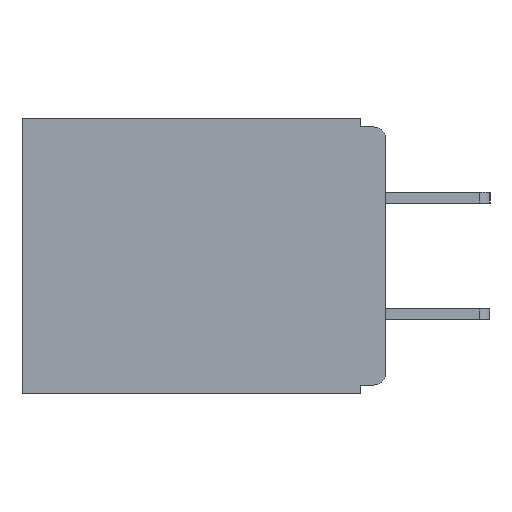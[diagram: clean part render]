
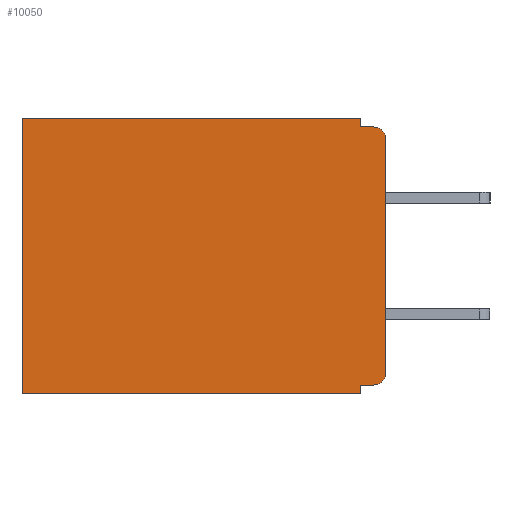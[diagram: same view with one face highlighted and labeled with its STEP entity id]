
A CAD part, left-side view. The second image highlights one B-rep face of the part: STEP entity #10050.
In plain terms, the highlighted planar face has unit normal (-1, 0, 0).
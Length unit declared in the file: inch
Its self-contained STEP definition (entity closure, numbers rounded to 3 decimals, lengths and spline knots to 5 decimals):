
#286 = LINE ( 'NONE', #6768, #24448 ) ;
#321 = DIRECTION ( 'NONE',  ( 0., 1., 0. ) ) ;
#664 = CARTESIAN_POINT ( 'NONE',  ( 0.3, 0., -0.33 ) ) ;
#1757 = CARTESIAN_POINT ( 'NONE',  ( 0.3, 0., -0.01 ) ) ;
#1906 = DIRECTION ( 'NONE',  ( 1., 0., 0. ) ) ;
#2193 = CARTESIAN_POINT ( 'NONE',  ( 0.3, 0.031, -0.32 ) ) ;
#2495 = LINE ( 'NONE', #664, #7075 ) ;
#2692 = DIRECTION ( 'NONE',  ( 0., 0., -1. ) ) ;
#2815 = CARTESIAN_POINT ( 'NONE',  ( 0.3, 0.437, -0.33 ) ) ;
#3931 = DIRECTION ( 'NONE',  ( 0., 0., -1. ) ) ;
#4431 = VECTOR ( 'NONE', #19743, 39.37008 ) ;
#6627 = CARTESIAN_POINT ( 'NONE',  ( 0.3, 0.015, -0.32 ) ) ;
#6768 = CARTESIAN_POINT ( 'NONE',  ( 0.3, 0., -0.33 ) ) ;
#7075 = VECTOR ( 'NONE', #2692, 39.37008 ) ;
#7215 = ORIENTED_EDGE ( 'NONE', *, *, #11535, .F. ) ;
#7394 = VECTOR ( 'NONE', #9188, 39.37008 ) ;
#7832 = EDGE_CURVE ( 'NONE', #14480, #10644, #13323, .T. ) ;
#7891 = VECTOR ( 'NONE', #321, 39.37008 ) ;
#8687 = DIRECTION ( 'NONE',  ( 0., 1., 0. ) ) ;
#9079 = VERTEX_POINT ( 'NONE', #23407 ) ;
#9143 = AXIS2_PLACEMENT_3D ( 'NONE', #13459, #1906, #15392 ) ;
#9188 = DIRECTION ( 'NONE',  ( 0., 0., -1. ) ) ;
#9227 = EDGE_CURVE ( 'NONE', #20354, #9079, #17417, .T. ) ;
#9714 = CARTESIAN_POINT ( 'NONE',  ( 0.3, 0.437, 0. ) ) ;
#10050 = ADVANCED_FACE ( 'NONE', ( #20315 ), #22793, .F. ) ;
#10409 = CARTESIAN_POINT ( 'NONE',  ( 0.3, 0., 0. ) ) ;
#10644 = VERTEX_POINT ( 'NONE', #9714 ) ;
#10676 = CARTESIAN_POINT ( 'NONE',  ( 0.3, 0.015, -0.305 ) ) ;
#10897 = LINE ( 'NONE', #11620, #20394 ) ;
#11111 = CARTESIAN_POINT ( 'NONE',  ( 0.3, 0.015, -0.025 ) ) ;
#11207 = VERTEX_POINT ( 'NONE', #22508 ) ;
#11514 = ORIENTED_EDGE ( 'NONE', *, *, #14341, .T. ) ;
#11535 = EDGE_CURVE ( 'NONE', #20855, #21771, #14666, .T. ) ;
#11620 = CARTESIAN_POINT ( 'NONE',  ( 0.3, 0.437, -0.33 ) ) ;
#11855 = EDGE_CURVE ( 'NONE', #18070, #24520, #23090, .T. ) ;
#12035 = CARTESIAN_POINT ( 'NONE',  ( 0.3, 0., -0.32 ) ) ;
#12287 = CARTESIAN_POINT ( 'NONE',  ( 0.3, 0.031, -0.33 ) ) ;
#12364 = DIRECTION ( 'NONE',  ( 0., 1., 0. ) ) ;
#12646 = DIRECTION ( 'NONE',  ( 0., 0., -1. ) ) ;
#12737 = VECTOR ( 'NONE', #12364, 39.37008 ) ;
#12825 = EDGE_CURVE ( 'NONE', #14480, #11207, #23047, .T. ) ;
#13076 = DIRECTION ( 'NONE',  ( 0., 0., -1. ) ) ;
#13110 = VECTOR ( 'NONE', #24518, 39.37008 ) ;
#13323 = LINE ( 'NONE', #10409, #12737 ) ;
#13459 = CARTESIAN_POINT ( 'NONE',  ( 0.3, 0., -0.33 ) ) ;
#14123 = ORIENTED_EDGE ( 'NONE', *, *, #14417, .F. ) ;
#14160 = CARTESIAN_POINT ( 'NONE',  ( 0.3, 0., -0.025 ) ) ;
#14341 = EDGE_CURVE ( 'NONE', #10644, #20374, #10897, .T. ) ;
#14417 = EDGE_CURVE ( 'NONE', #20354, #20855, #22397, .T. ) ;
#14480 = VERTEX_POINT ( 'NONE', #15953 ) ;
#14666 = LINE ( 'NONE', #17859, #4431 ) ;
#14939 = CARTESIAN_POINT ( 'NONE',  ( 0.3, 0.031, 0. ) ) ;
#15339 = ORIENTED_EDGE ( 'NONE', *, *, #24354, .F. ) ;
#15392 = DIRECTION ( 'NONE',  ( 0., 0., -1. ) ) ;
#15764 = AXIS2_PLACEMENT_3D ( 'NONE', #10676, #23812, #12646 ) ;
#15953 = CARTESIAN_POINT ( 'NONE',  ( 0.3, 0.031, 0. ) ) ;
#17133 = ORIENTED_EDGE ( 'NONE', *, *, #9227, .T. ) ;
#17417 = CIRCLE ( 'NONE', #15764, 0.015 ) ;
#17859 = CARTESIAN_POINT ( 'NONE',  ( 0.3, 0.031, -0.33 ) ) ;
#18070 = VERTEX_POINT ( 'NONE', #14160 ) ;
#18104 = LINE ( 'NONE', #1757, #13110 ) ;
#19134 = EDGE_CURVE ( 'NONE', #21771, #20374, #286, .T. ) ;
#19446 = EDGE_CURVE ( 'NONE', #11207, #24520, #18104, .T. ) ;
#19743 = DIRECTION ( 'NONE',  ( 0., 0., -1. ) ) ;
#19756 = ORIENTED_EDGE ( 'NONE', *, *, #11855, .T. ) ;
#20215 = ORIENTED_EDGE ( 'NONE', *, *, #7832, .T. ) ;
#20315 = FACE_OUTER_BOUND ( 'NONE', #22550, .T. ) ;
#20354 = VERTEX_POINT ( 'NONE', #6627 ) ;
#20374 = VERTEX_POINT ( 'NONE', #2815 ) ;
#20394 = VECTOR ( 'NONE', #3931, 39.37008 ) ;
#20520 = ORIENTED_EDGE ( 'NONE', *, *, #12825, .F. ) ;
#20855 = VERTEX_POINT ( 'NONE', #2193 ) ;
#20920 = ORIENTED_EDGE ( 'NONE', *, *, #19134, .F. ) ;
#21771 = VERTEX_POINT ( 'NONE', #12287 ) ;
#22033 = AXIS2_PLACEMENT_3D ( 'NONE', #11111, #24200, #13076 ) ;
#22185 = CARTESIAN_POINT ( 'NONE',  ( 0.3, 0.015, -0.01 ) ) ;
#22337 = ORIENTED_EDGE ( 'NONE', *, *, #19446, .F. ) ;
#22397 = LINE ( 'NONE', #12035, #7891 ) ;
#22508 = CARTESIAN_POINT ( 'NONE',  ( 0.3, 0.031, -0.01 ) ) ;
#22550 = EDGE_LOOP ( 'NONE', ( #15339, #19756, #22337, #20520, #20215, #11514, #20920, #7215, #14123, #17133 ) ) ;
#22793 = PLANE ( 'NONE',  #9143 ) ;
#23047 = LINE ( 'NONE', #14939, #7394 ) ;
#23090 = CIRCLE ( 'NONE', #22033, 0.015 ) ;
#23407 = CARTESIAN_POINT ( 'NONE',  ( 0.3, 0., -0.305 ) ) ;
#23812 = DIRECTION ( 'NONE',  ( -1., 0., 0. ) ) ;
#24200 = DIRECTION ( 'NONE',  ( -1., 0., 0. ) ) ;
#24354 = EDGE_CURVE ( 'NONE', #18070, #9079, #2495, .T. ) ;
#24448 = VECTOR ( 'NONE', #8687, 39.37008 ) ;
#24518 = DIRECTION ( 'NONE',  ( 0., -1., 0. ) ) ;
#24520 = VERTEX_POINT ( 'NONE', #22185 ) ;
